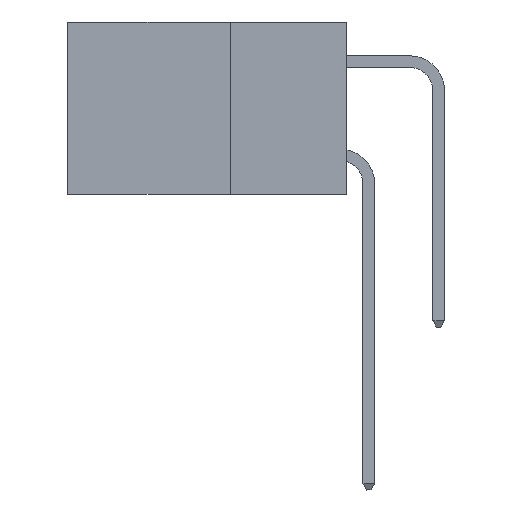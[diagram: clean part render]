
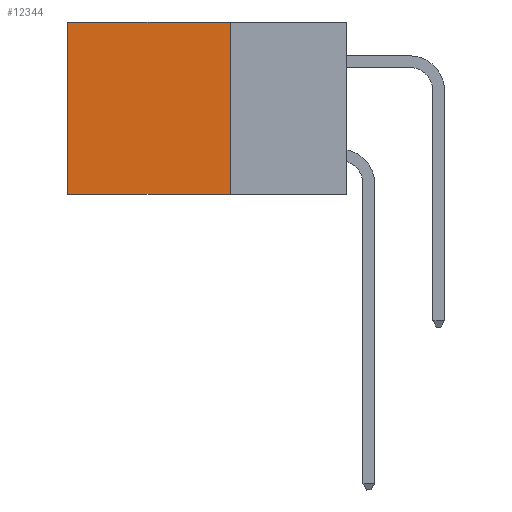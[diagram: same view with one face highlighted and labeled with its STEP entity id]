
A CAD part, left-side view. The second image highlights one B-rep face of the part: STEP entity #12344.
In plain terms, the highlighted planar face has unit normal (-1, 0, 0).
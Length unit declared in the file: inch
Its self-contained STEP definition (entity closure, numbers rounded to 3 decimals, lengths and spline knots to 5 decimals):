
#2478 = CARTESIAN_POINT ( 'NONE',  ( 0.2875, 0.25, -0.37 ) ) ;
#2588 = DIRECTION ( 'NONE',  ( 0., 1., 0. ) ) ;
#3034 = FACE_OUTER_BOUND ( 'NONE', #8786, .T. ) ;
#3095 = DIRECTION ( 'NONE',  ( 0., 0., -1. ) ) ;
#3974 = LINE ( 'NONE', #8931, #31635 ) ;
#4828 = ORIENTED_EDGE ( 'NONE', *, *, #26723, .F. ) ;
#6487 = CARTESIAN_POINT ( 'NONE',  ( 0.2875, 0.25, -0.37 ) ) ;
#6541 = EDGE_CURVE ( 'NONE', #28930, #14347, #16866, .T. ) ;
#7631 = CARTESIAN_POINT ( 'NONE',  ( 0.2875, 0.6, 0. ) ) ;
#7849 = LINE ( 'NONE', #23677, #21959 ) ;
#7854 = DIRECTION ( 'NONE',  ( 0., 0., -1. ) ) ;
#8285 = DIRECTION ( 'NONE',  ( 0., 0., -1. ) ) ;
#8786 = EDGE_LOOP ( 'NONE', ( #13076, #4828, #15471, #30419 ) ) ;
#8931 = CARTESIAN_POINT ( 'NONE',  ( 0.2875, 0.25, 0. ) ) ;
#10153 = VERTEX_POINT ( 'NONE', #6487 ) ;
#11529 = DIRECTION ( 'NONE',  ( 0., 1., 0. ) ) ;
#12344 = ADVANCED_FACE ( 'NONE', ( #3034 ), #20787, .F. ) ;
#13076 = ORIENTED_EDGE ( 'NONE', *, *, #6541, .T. ) ;
#14347 = VERTEX_POINT ( 'NONE', #31818 ) ;
#15407 = CARTESIAN_POINT ( 'NONE',  ( 0.2875, 0.25, 0. ) ) ;
#15471 = ORIENTED_EDGE ( 'NONE', *, *, #18337, .F. ) ;
#15712 = VECTOR ( 'NONE', #2588, 39.37008 ) ;
#16866 = LINE ( 'NONE', #7631, #26417 ) ;
#18337 = EDGE_CURVE ( 'NONE', #25102, #10153, #7849, .T. ) ;
#20787 = PLANE ( 'NONE',  #31313 ) ;
#21213 = CARTESIAN_POINT ( 'NONE',  ( 0.2875, 0.6, 0. ) ) ;
#21959 = VECTOR ( 'NONE', #8285, 39.37008 ) ;
#22544 = LINE ( 'NONE', #2478, #15712 ) ;
#22717 = EDGE_CURVE ( 'NONE', #25102, #28930, #3974, .T. ) ;
#23677 = CARTESIAN_POINT ( 'NONE',  ( 0.2875, 0.25, 0. ) ) ;
#25102 = VERTEX_POINT ( 'NONE', #15407 ) ;
#26417 = VECTOR ( 'NONE', #7854, 39.37008 ) ;
#26723 = EDGE_CURVE ( 'NONE', #10153, #14347, #22544, .T. ) ;
#28930 = VERTEX_POINT ( 'NONE', #21213 ) ;
#28992 = DIRECTION ( 'NONE',  ( 1., 0., 0. ) ) ;
#30419 = ORIENTED_EDGE ( 'NONE', *, *, #22717, .T. ) ;
#31046 = CARTESIAN_POINT ( 'NONE',  ( 0.2875, 0.25, 0. ) ) ;
#31313 = AXIS2_PLACEMENT_3D ( 'NONE', #31046, #28992, #3095 ) ;
#31635 = VECTOR ( 'NONE', #11529, 39.37008 ) ;
#31818 = CARTESIAN_POINT ( 'NONE',  ( 0.2875, 0.6, -0.37 ) ) ;
